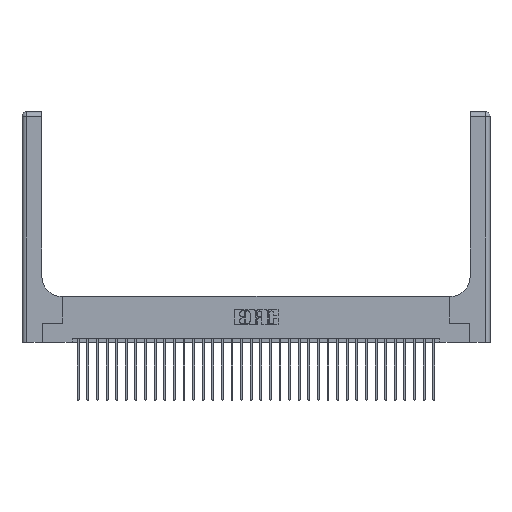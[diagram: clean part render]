
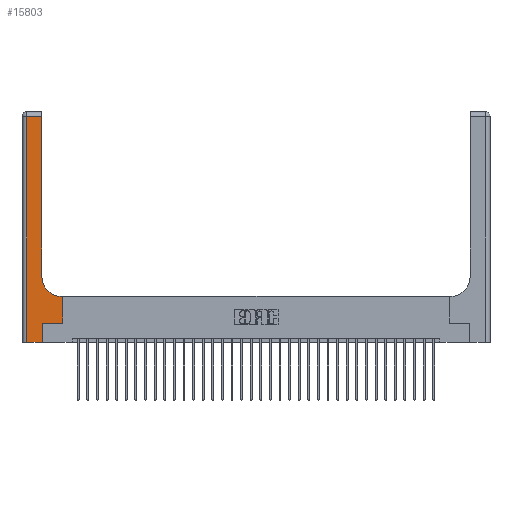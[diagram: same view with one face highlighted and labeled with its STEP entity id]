
A CAD part, top view. The second image highlights one B-rep face of the part: STEP entity #15803.
In plain terms, the highlighted planar face has unit normal (0, 0, 1).
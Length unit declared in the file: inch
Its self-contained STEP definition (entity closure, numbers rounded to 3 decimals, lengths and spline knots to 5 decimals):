
#43 = DIRECTION ( 'NONE',  ( 0., -1., 0. ) ) ;
#109 = DIRECTION ( 'NONE',  ( 0., 0., -1. ) ) ;
#327 = DIRECTION ( 'NONE',  ( -1., 0., 0. ) ) ;
#369 = VECTOR ( 'NONE', #21313, 39.37008 ) ;
#1288 = VECTOR ( 'NONE', #43, 39.37008 ) ;
#1756 = CARTESIAN_POINT ( 'NONE',  ( 0.528, 0.6, 0.37 ) ) ;
#1935 = EDGE_CURVE ( 'NONE', #8640, #3415, #19725, .T. ) ;
#2118 = CARTESIAN_POINT ( 'NONE',  ( 0.265, 0.25, 0.37 ) ) ;
#2371 = PLANE ( 'NONE',  #18255 ) ;
#2923 = EDGE_CURVE ( 'NONE', #24088, #10153, #29090, .T. ) ;
#3009 = DIRECTION ( 'NONE',  ( 0., 1., 0. ) ) ;
#3415 = VERTEX_POINT ( 'NONE', #22325 ) ;
#4085 = EDGE_CURVE ( 'NONE', #24311, #13177, #26133, .T. ) ;
#5032 = CARTESIAN_POINT ( 'NONE',  ( 0.26, 3., 0.37 ) ) ;
#5336 = ORIENTED_EDGE ( 'NONE', *, *, #1935, .T. ) ;
#5529 = CARTESIAN_POINT ( 'NONE',  ( 0.265, 0., 0.37 ) ) ;
#5647 = CARTESIAN_POINT ( 'NONE',  ( 0.06, 2.94, 0.37 ) ) ;
#6442 = CARTESIAN_POINT ( 'NONE',  ( 0.06, 0., 0.37 ) ) ;
#8640 = VERTEX_POINT ( 'NONE', #10362 ) ;
#9029 = DIRECTION ( 'NONE',  ( -1., 0., 0. ) ) ;
#9051 = LINE ( 'NONE', #2118, #26009 ) ;
#10153 = VERTEX_POINT ( 'NONE', #1756 ) ;
#10218 = ORIENTED_EDGE ( 'NONE', *, *, #4085, .T. ) ;
#10362 = CARTESIAN_POINT ( 'NONE',  ( 0.51, 0.6, 0.37 ) ) ;
#11270 = VECTOR ( 'NONE', #3009, 39.37008 ) ;
#11383 = LINE ( 'NONE', #30529, #22294 ) ;
#11914 = ORIENTED_EDGE ( 'NONE', *, *, #22605, .T. ) ;
#12168 = AXIS2_PLACEMENT_3D ( 'NONE', #19301, #109, #21804 ) ;
#12190 = ORIENTED_EDGE ( 'NONE', *, *, #25366, .T. ) ;
#12904 = ORIENTED_EDGE ( 'NONE', *, *, #20188, .T. ) ;
#13177 = VERTEX_POINT ( 'NONE', #6442 ) ;
#13317 = VECTOR ( 'NONE', #14642, 39.37008 ) ;
#13872 = CARTESIAN_POINT ( 'NONE',  ( 0.528, 0.25, 0.37 ) ) ;
#13884 = VERTEX_POINT ( 'NONE', #16567 ) ;
#13929 = DIRECTION ( 'NONE',  ( 1., 0., 0. ) ) ;
#14575 = ORIENTED_EDGE ( 'NONE', *, *, #25692, .T. ) ;
#14642 = DIRECTION ( 'NONE',  ( 0., 1., 0. ) ) ;
#15803 = ADVANCED_FACE ( 'NONE', ( #26414 ), #2371, .F. ) ;
#15817 = LINE ( 'NONE', #23527, #369 ) ;
#16555 = CARTESIAN_POINT ( 'NONE',  ( 0.06, 3., 0.37 ) ) ;
#16567 = CARTESIAN_POINT ( 'NONE',  ( 0.26, 2.94, 0.37 ) ) ;
#16846 = LINE ( 'NONE', #5032, #13317 ) ;
#17006 = DIRECTION ( 'NONE',  ( 0., 0., -1. ) ) ;
#17402 = VERTEX_POINT ( 'NONE', #5529 ) ;
#18255 = AXIS2_PLACEMENT_3D ( 'NONE', #19518, #17006, #327 ) ;
#18552 = DIRECTION ( 'NONE',  ( 1., 0., 0. ) ) ;
#19062 = VERTEX_POINT ( 'NONE', #19070 ) ;
#19070 = CARTESIAN_POINT ( 'NONE',  ( 0.265, 0.25, 0.37 ) ) ;
#19301 = CARTESIAN_POINT ( 'NONE',  ( 0.51, 0.85, 0.37 ) ) ;
#19351 = EDGE_LOOP ( 'NONE', ( #27838, #11914, #10218, #14575, #12190, #12904, #24478, #22262, #5336 ) ) ;
#19383 = VECTOR ( 'NONE', #18552, 39.37008 ) ;
#19518 = CARTESIAN_POINT ( 'NONE',  ( 0., 3., 0.37 ) ) ;
#19725 = CIRCLE ( 'NONE', #12168, 0.25 ) ;
#20188 = EDGE_CURVE ( 'NONE', #19062, #24088, #9051, .T. ) ;
#21313 = DIRECTION ( 'NONE',  ( -1., 0., 0. ) ) ;
#21804 = DIRECTION ( 'NONE',  ( 1., 0., 0. ) ) ;
#21846 = CARTESIAN_POINT ( 'NONE',  ( 0.265, 0., 0.37 ) ) ;
#22262 = ORIENTED_EDGE ( 'NONE', *, *, #29456, .T. ) ;
#22294 = VECTOR ( 'NONE', #9029, 39.37008 ) ;
#22325 = CARTESIAN_POINT ( 'NONE',  ( 0.26, 0.85, 0.37 ) ) ;
#22605 = EDGE_CURVE ( 'NONE', #13884, #24311, #11383, .T. ) ;
#23527 = CARTESIAN_POINT ( 'NONE',  ( 0.26, 0.6, 0.37 ) ) ;
#24088 = VERTEX_POINT ( 'NONE', #13872 ) ;
#24232 = EDGE_CURVE ( 'NONE', #3415, #13884, #16846, .T. ) ;
#24311 = VERTEX_POINT ( 'NONE', #5647 ) ;
#24478 = ORIENTED_EDGE ( 'NONE', *, *, #2923, .T. ) ;
#24815 = DIRECTION ( 'NONE',  ( 0., 1., 0. ) ) ;
#25366 = EDGE_CURVE ( 'NONE', #17402, #19062, #27017, .T. ) ;
#25692 = EDGE_CURVE ( 'NONE', #13177, #17402, #30591, .T. ) ;
#26009 = VECTOR ( 'NONE', #13929, 39.37008 ) ;
#26133 = LINE ( 'NONE', #16555, #1288 ) ;
#26414 = FACE_OUTER_BOUND ( 'NONE', #19351, .T. ) ;
#26739 = CARTESIAN_POINT ( 'NONE',  ( 0.528, 0.25, 0.37 ) ) ;
#27017 = LINE ( 'NONE', #21846, #29390 ) ;
#27838 = ORIENTED_EDGE ( 'NONE', *, *, #24232, .T. ) ;
#29090 = LINE ( 'NONE', #26739, #11270 ) ;
#29390 = VECTOR ( 'NONE', #24815, 39.37008 ) ;
#29456 = EDGE_CURVE ( 'NONE', #10153, #8640, #15817, .T. ) ;
#30434 = CARTESIAN_POINT ( 'NONE',  ( 0., 0., 0.37 ) ) ;
#30529 = CARTESIAN_POINT ( 'NONE',  ( 0., 2.94, 0.37 ) ) ;
#30591 = LINE ( 'NONE', #30434, #19383 ) ;
